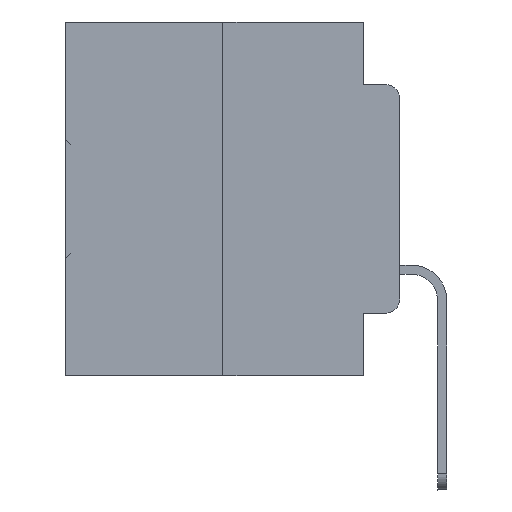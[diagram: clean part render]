
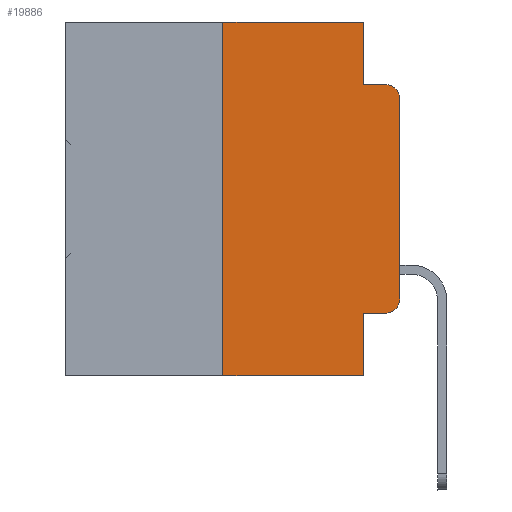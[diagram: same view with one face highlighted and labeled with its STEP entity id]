
A CAD part, left-side view. The second image highlights one B-rep face of the part: STEP entity #19886.
In plain terms, the highlighted planar face has unit normal (-1, 0, 0).
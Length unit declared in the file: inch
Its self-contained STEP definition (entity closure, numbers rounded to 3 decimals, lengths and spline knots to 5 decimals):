
#918 = DIRECTION ( 'NONE',  ( 0., -1., 0. ) ) ;
#1140 = CARTESIAN_POINT ( 'NONE',  ( 0., 0.25, 0. ) ) ;
#1176 = VECTOR ( 'NONE', #2891, 39.37008 ) ;
#1203 = FACE_OUTER_BOUND ( 'NONE', #21293, .T. ) ;
#1250 = CARTESIAN_POINT ( 'NONE',  ( 0., 0.051, -0.4115 ) ) ;
#2587 = VECTOR ( 'NONE', #14157, 39.37008 ) ;
#2891 = DIRECTION ( 'NONE',  ( 0., -1., 0. ) ) ;
#3121 = CARTESIAN_POINT ( 'NONE',  ( 0., 0.25, -0.5 ) ) ;
#3182 = AXIS2_PLACEMENT_3D ( 'NONE', #13918, #11405, #16275 ) ;
#3637 = DIRECTION ( 'NONE',  ( 0., 0., -1. ) ) ;
#3743 = VECTOR ( 'NONE', #3637, 39.37008 ) ;
#3947 = CARTESIAN_POINT ( 'NONE',  ( 0., 0.473, 0. ) ) ;
#4658 = ORIENTED_EDGE ( 'NONE', *, *, #17234, .T. ) ;
#5248 = ORIENTED_EDGE ( 'NONE', *, *, #30443, .T. ) ;
#6066 = CARTESIAN_POINT ( 'NONE',  ( 0., 0.051, 0. ) ) ;
#6313 = CARTESIAN_POINT ( 'NONE',  ( 0., 0.25, 0. ) ) ;
#6429 = DIRECTION ( 'NONE',  ( -1., 0., 0. ) ) ;
#6645 = LINE ( 'NONE', #6313, #15414 ) ;
#7027 = DIRECTION ( 'NONE',  ( -1., 0., 0. ) ) ;
#7747 = LINE ( 'NONE', #23177, #1176 ) ;
#7757 = CARTESIAN_POINT ( 'NONE',  ( 0., 0., -0.1085 ) ) ;
#8087 = CARTESIAN_POINT ( 'NONE',  ( 0., 0., -0.3915 ) ) ;
#8383 = VECTOR ( 'NONE', #31807, 39.37008 ) ;
#8530 = CARTESIAN_POINT ( 'NONE',  ( 0., 0.02, -0.0885 ) ) ;
#9385 = VECTOR ( 'NONE', #16282, 39.37008 ) ;
#10153 = EDGE_CURVE ( 'NONE', #11986, #22275, #7747, .T. ) ;
#11154 = ORIENTED_EDGE ( 'NONE', *, *, #20614, .F. ) ;
#11405 = DIRECTION ( 'NONE',  ( 1., 0., 0. ) ) ;
#11484 = LINE ( 'NONE', #3947, #2587 ) ;
#11986 = VERTEX_POINT ( 'NONE', #31922 ) ;
#12112 = ORIENTED_EDGE ( 'NONE', *, *, #13924, .T. ) ;
#12596 = ORIENTED_EDGE ( 'NONE', *, *, #19103, .F. ) ;
#13067 = AXIS2_PLACEMENT_3D ( 'NONE', #22287, #7027, #27839 ) ;
#13221 = EDGE_CURVE ( 'NONE', #32461, #28557, #31961, .T. ) ;
#13679 = CARTESIAN_POINT ( 'NONE',  ( 0., 0.051, 0. ) ) ;
#13918 = CARTESIAN_POINT ( 'NONE',  ( 0., 0.473, 0. ) ) ;
#13924 = EDGE_CURVE ( 'NONE', #28557, #32433, #15745, .T. ) ;
#14093 = ORIENTED_EDGE ( 'NONE', *, *, #19533, .T. ) ;
#14157 = DIRECTION ( 'NONE',  ( 0., -1., 0. ) ) ;
#14360 = AXIS2_PLACEMENT_3D ( 'NONE', #29424, #6429, #26891 ) ;
#14385 = CIRCLE ( 'NONE', #14360, 0.02 ) ;
#15414 = VECTOR ( 'NONE', #31998, 39.37008 ) ;
#15745 = CIRCLE ( 'NONE', #13067, 0.02 ) ;
#15959 = CARTESIAN_POINT ( 'NONE',  ( 0., 0.051, 0. ) ) ;
#16131 = ORIENTED_EDGE ( 'NONE', *, *, #13221, .T. ) ;
#16275 = DIRECTION ( 'NONE',  ( 0., 0., -1. ) ) ;
#16282 = DIRECTION ( 'NONE',  ( 0., 0., -1. ) ) ;
#16714 = CARTESIAN_POINT ( 'NONE',  ( 0., 0., 0. ) ) ;
#17234 = EDGE_CURVE ( 'NONE', #32433, #32210, #32188, .T. ) ;
#17756 = CARTESIAN_POINT ( 'NONE',  ( 0., 0.051, -0.5 ) ) ;
#19074 = DIRECTION ( 'NONE',  ( 0., 0., 1. ) ) ;
#19103 = EDGE_CURVE ( 'NONE', #28840, #25356, #11484, .T. ) ;
#19297 = PLANE ( 'NONE',  #3182 ) ;
#19533 = EDGE_CURVE ( 'NONE', #32210, #22275, #14385, .T. ) ;
#19886 = ADVANCED_FACE ( 'NONE', ( #1203 ), #19297, .F. ) ;
#20547 = VECTOR ( 'NONE', #918, 39.37008 ) ;
#20614 = EDGE_CURVE ( 'NONE', #25356, #11986, #27188, .T. ) ;
#21293 = EDGE_LOOP ( 'NONE', ( #4658, #14093, #30989, #11154, #12596, #29042, #5248, #31560, #16131, #12112 ) ) ;
#21997 = CARTESIAN_POINT ( 'NONE',  ( 0., 0.051, -0.4115 ) ) ;
#22275 = VERTEX_POINT ( 'NONE', #8530 ) ;
#22287 = CARTESIAN_POINT ( 'NONE',  ( 0., 0.02, -0.3915 ) ) ;
#22800 = EDGE_CURVE ( 'NONE', #30535, #28840, #6645, .T. ) ;
#23177 = CARTESIAN_POINT ( 'NONE',  ( 0., 0.051, -0.0885 ) ) ;
#23893 = LINE ( 'NONE', #29126, #8383 ) ;
#24707 = EDGE_CURVE ( 'NONE', #32461, #33058, #32003, .T. ) ;
#25356 = VERTEX_POINT ( 'NONE', #15959 ) ;
#25613 = VECTOR ( 'NONE', #19074, 39.37008 ) ;
#26891 = DIRECTION ( 'NONE',  ( 0., 0., -1. ) ) ;
#27188 = LINE ( 'NONE', #6066, #9385 ) ;
#27839 = DIRECTION ( 'NONE',  ( 0., 0., -1. ) ) ;
#28557 = VERTEX_POINT ( 'NONE', #30193 ) ;
#28840 = VERTEX_POINT ( 'NONE', #1140 ) ;
#29042 = ORIENTED_EDGE ( 'NONE', *, *, #22800, .F. ) ;
#29126 = CARTESIAN_POINT ( 'NONE',  ( 0., 0.473, -0.5 ) ) ;
#29424 = CARTESIAN_POINT ( 'NONE',  ( 0., 0.02, -0.1085 ) ) ;
#30193 = CARTESIAN_POINT ( 'NONE',  ( 0., 0.02, -0.4115 ) ) ;
#30443 = EDGE_CURVE ( 'NONE', #30535, #33058, #23893, .T. ) ;
#30535 = VERTEX_POINT ( 'NONE', #3121 ) ;
#30989 = ORIENTED_EDGE ( 'NONE', *, *, #10153, .F. ) ;
#31560 = ORIENTED_EDGE ( 'NONE', *, *, #24707, .F. ) ;
#31807 = DIRECTION ( 'NONE',  ( 0., -1., 0. ) ) ;
#31922 = CARTESIAN_POINT ( 'NONE',  ( 0., 0.051, -0.0885 ) ) ;
#31961 = LINE ( 'NONE', #1250, #20547 ) ;
#31998 = DIRECTION ( 'NONE',  ( 0., 0., 1. ) ) ;
#32003 = LINE ( 'NONE', #13679, #3743 ) ;
#32188 = LINE ( 'NONE', #16714, #25613 ) ;
#32210 = VERTEX_POINT ( 'NONE', #7757 ) ;
#32433 = VERTEX_POINT ( 'NONE', #8087 ) ;
#32461 = VERTEX_POINT ( 'NONE', #21997 ) ;
#33058 = VERTEX_POINT ( 'NONE', #17756 ) ;
